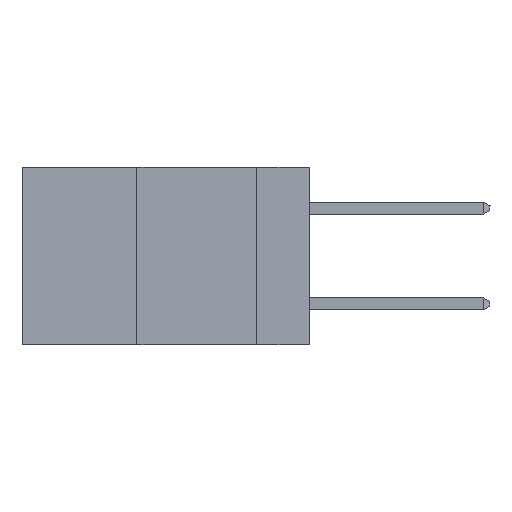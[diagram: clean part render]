
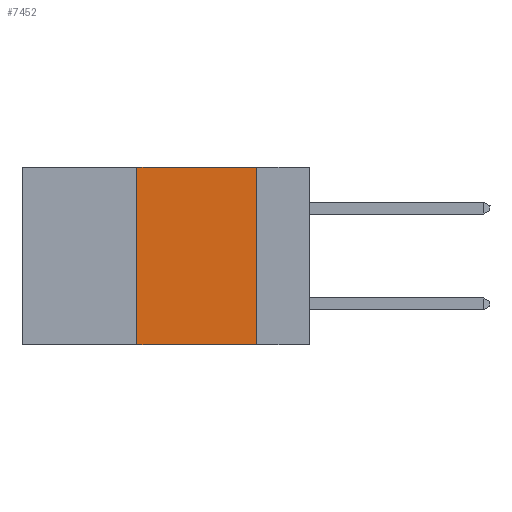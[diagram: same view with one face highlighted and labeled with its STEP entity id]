
A CAD part, left-side view. The second image highlights one B-rep face of the part: STEP entity #7452.
In plain terms, the highlighted planar face has unit normal (-1, 0, 0).
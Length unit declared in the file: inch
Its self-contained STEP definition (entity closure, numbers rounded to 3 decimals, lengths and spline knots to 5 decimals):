
#557 = CARTESIAN_POINT ( 'NONE',  ( 0., 0.6, 0. ) ) ;
#719 = DIRECTION ( 'NONE',  ( 1., 0., 0. ) ) ;
#1257 = VERTEX_POINT ( 'NONE', #8229 ) ;
#1489 = DIRECTION ( 'NONE',  ( 0., -1., 0. ) ) ;
#1778 = PLANE ( 'NONE',  #10597 ) ;
#2057 = ORIENTED_EDGE ( 'NONE', *, *, #2955, .F. ) ;
#2538 = ORIENTED_EDGE ( 'NONE', *, *, #6756, .F. ) ;
#2789 = LINE ( 'NONE', #6764, #9010 ) ;
#2863 = VECTOR ( 'NONE', #6163, 39.37008 ) ;
#2955 = EDGE_CURVE ( 'NONE', #1257, #3085, #4960, .T. ) ;
#3085 = VERTEX_POINT ( 'NONE', #9160 ) ;
#3680 = DIRECTION ( 'NONE',  ( 0., -1., 0. ) ) ;
#3702 = EDGE_CURVE ( 'NONE', #1257, #10780, #6717, .T. ) ;
#3737 = CARTESIAN_POINT ( 'NONE',  ( 0., 0.11, 0. ) ) ;
#3937 = DIRECTION ( 'NONE',  ( 0., 0., -1. ) ) ;
#4637 = DIRECTION ( 'NONE',  ( 0., 0., -1. ) ) ;
#4960 = LINE ( 'NONE', #10832, #2863 ) ;
#5180 = VERTEX_POINT ( 'NONE', #3737 ) ;
#6089 = EDGE_CURVE ( 'NONE', #3085, #5180, #11664, .T. ) ;
#6163 = DIRECTION ( 'NONE',  ( 0., 0., 1. ) ) ;
#6505 = CARTESIAN_POINT ( 'NONE',  ( 0., 0.6, 0. ) ) ;
#6717 = LINE ( 'NONE', #12138, #9657 ) ;
#6756 = EDGE_CURVE ( 'NONE', #5180, #10780, #2789, .T. ) ;
#6764 = CARTESIAN_POINT ( 'NONE',  ( 0., 0.11, 0. ) ) ;
#7452 = ADVANCED_FACE ( 'NONE', ( #9851 ), #1778, .F. ) ;
#7526 = ORIENTED_EDGE ( 'NONE', *, *, #6089, .F. ) ;
#8229 = CARTESIAN_POINT ( 'NONE',  ( 0., 0.36, -0.37 ) ) ;
#9010 = VECTOR ( 'NONE', #3937, 39.37008 ) ;
#9160 = CARTESIAN_POINT ( 'NONE',  ( 0., 0.36, 0. ) ) ;
#9162 = VECTOR ( 'NONE', #1489, 39.37008 ) ;
#9277 = EDGE_LOOP ( 'NONE', ( #2538, #7526, #2057, #10272 ) ) ;
#9657 = VECTOR ( 'NONE', #3680, 39.37008 ) ;
#9851 = FACE_OUTER_BOUND ( 'NONE', #9277, .T. ) ;
#10008 = CARTESIAN_POINT ( 'NONE',  ( 0., 0.11, -0.37 ) ) ;
#10272 = ORIENTED_EDGE ( 'NONE', *, *, #3702, .T. ) ;
#10597 = AXIS2_PLACEMENT_3D ( 'NONE', #6505, #719, #4637 ) ;
#10780 = VERTEX_POINT ( 'NONE', #10008 ) ;
#10832 = CARTESIAN_POINT ( 'NONE',  ( 0., 0.36, 0. ) ) ;
#11664 = LINE ( 'NONE', #557, #9162 ) ;
#12138 = CARTESIAN_POINT ( 'NONE',  ( 0., 0.6, -0.37 ) ) ;
